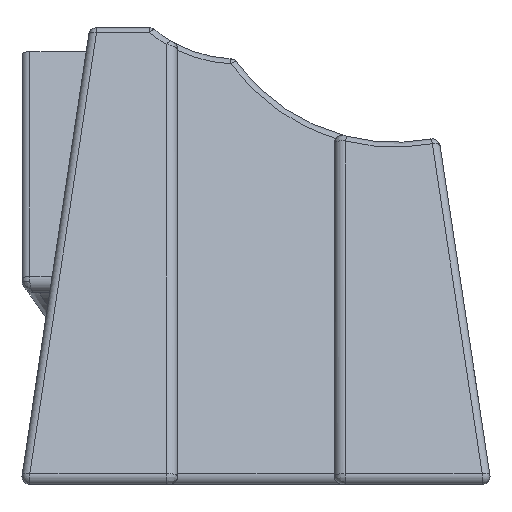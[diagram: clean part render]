
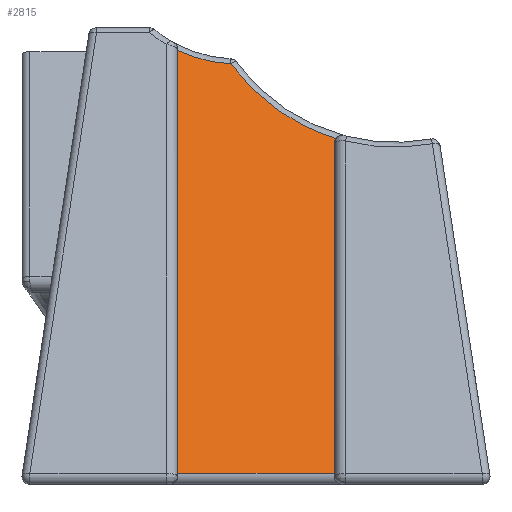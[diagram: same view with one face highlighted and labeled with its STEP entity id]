
A CAD part, top view. The second image highlights one B-rep face of the part: STEP entity #2815.
In plain terms, the highlighted planar face has unit normal (0, 0.375, 0.927).
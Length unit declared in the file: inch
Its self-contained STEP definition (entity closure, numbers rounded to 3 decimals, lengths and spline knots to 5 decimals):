
#331=FACE_OUTER_BOUND('',#506,.T.);
#506=EDGE_LOOP('',(#2360,#2361,#2362,#2363,#2364,#2365));
#724=ELLIPSE('',#3077,0.28042,0.26);
#725=ELLIPSE('',#3079,0.01079,0.01);
#745=ELLIPSE('',#3141,0.18975,0.17593);
#859=LINE('',#5194,#1026);
#860=LINE('',#5198,#1027);
#884=LINE('',#5682,#1051);
#1026=VECTOR('',#3707,0.3937);
#1027=VECTOR('',#3712,0.3937);
#1051=VECTOR('',#3854,0.3937);
#1259=VERTEX_POINT('',#5173);
#1260=VERTEX_POINT('',#5175);
#1261=VERTEX_POINT('',#5188);
#1262=VERTEX_POINT('',#5193);
#1263=VERTEX_POINT('',#5197);
#1298=VERTEX_POINT('',#5680);
#1600=EDGE_CURVE('',#1259,#1260,#724,.T.);
#1604=EDGE_CURVE('',#1260,#1261,#725,.T.);
#1605=EDGE_CURVE('',#1262,#1261,#859,.T.);
#1607=EDGE_CURVE('',#1262,#1263,#860,.T.);
#1676=EDGE_CURVE('',#1298,#1259,#745,.T.);
#1677=EDGE_CURVE('',#1263,#1298,#884,.T.);
#2360=ORIENTED_EDGE('',*,*,#1607,.F.);
#2361=ORIENTED_EDGE('',*,*,#1605,.T.);
#2362=ORIENTED_EDGE('',*,*,#1604,.F.);
#2363=ORIENTED_EDGE('',*,*,#1600,.F.);
#2364=ORIENTED_EDGE('',*,*,#1676,.F.);
#2365=ORIENTED_EDGE('',*,*,#1677,.F.);
#2678=PLANE('',#3140);
#2815=ADVANCED_FACE('',(#331),#2678,.F.);
#3077=AXIS2_PLACEMENT_3D('',#5176,#3697,#3698);
#3079=AXIS2_PLACEMENT_3D('',#5191,#3703,#3704);
#3140=AXIS2_PLACEMENT_3D('',#5679,#3850,#3851);
#3141=AXIS2_PLACEMENT_3D('',#5681,#3852,#3853);
#3697=DIRECTION('center_axis',(0.,0.375,
0.927));
#3698=DIRECTION('ref_axis',(0.,-0.927,0.375));
#3703=DIRECTION('center_axis',(0.,0.375,
0.927));
#3704=DIRECTION('ref_axis',(0.,0.927,-0.375));
#3707=DIRECTION('',(0.,0.927,-0.375));
#3712=DIRECTION('',(-1.,0.,0.));
#3850=DIRECTION('center_axis',(0.,-0.375,
-0.927));
#3851=DIRECTION('ref_axis',(-1.,0.,0.));
#3852=DIRECTION('center_axis',(0.,0.375,
0.927));
#3853=DIRECTION('ref_axis',(0.,-0.927,0.375));
#3854=DIRECTION('',(0.,0.927,-0.375));
#5173=CARTESIAN_POINT('',(-0.24425,0.28992,-0.13331));
#5175=CARTESIAN_POINT('',(-0.10998,0.19469,-0.09484));
#5176=CARTESIAN_POINT('Origin',(-0.03445,0.44348,-0.19536));
#5188=CARTESIAN_POINT('',(-0.112,0.18866,-0.0924));
#5191=CARTESIAN_POINT('Origin',(-0.102,0.18866,-0.0924));
#5193=CARTESIAN_POINT('',(-0.112,-0.23299,0.07796));
#5194=CARTESIAN_POINT('',(-0.112,-0.26963,0.09276));
#5197=CARTESIAN_POINT('',(-0.312,-0.23299,0.07796));
#5198=CARTESIAN_POINT('',(-0.056,-0.23299,0.07796));
#5679=CARTESIAN_POINT('Origin',(-0.112,-0.26963,0.09276));
#5680=CARTESIAN_POINT('',(-0.312,0.30702,-0.14022));
#5681=CARTESIAN_POINT('Origin',(-0.23592,0.46565,-0.20431));
#5682=CARTESIAN_POINT('',(-0.312,-0.26963,0.09276));
